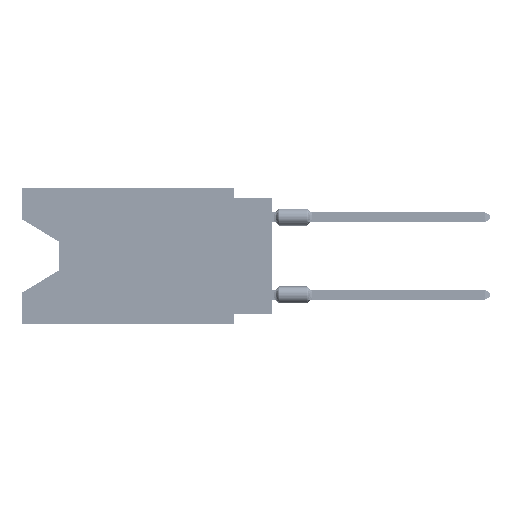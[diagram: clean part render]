
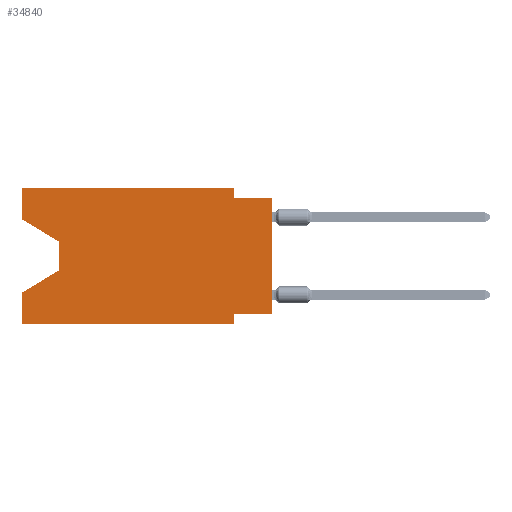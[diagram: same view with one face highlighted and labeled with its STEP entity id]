
A CAD part, left-side view. The second image highlights one B-rep face of the part: STEP entity #34840.
In plain terms, the highlighted planar face has unit normal (-1, 0, 0).
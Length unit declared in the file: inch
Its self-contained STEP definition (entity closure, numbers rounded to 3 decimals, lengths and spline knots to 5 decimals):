
#2917 = EDGE_CURVE ( 'NONE', #40746, #31872, #32700, .T. ) ;
#4210 = DIRECTION ( 'NONE',  ( 0., -1., 0. ) ) ;
#5944 = EDGE_CURVE ( 'NONE', #54752, #25376, #94050, .T. ) ;
#7796 = VECTOR ( 'NONE', #87289, 39.37008 ) ;
#8066 = LINE ( 'NONE', #54442, #36080 ) ;
#8804 = VECTOR ( 'NONE', #32441, 39.37008 ) ;
#9077 = AXIS2_PLACEMENT_3D ( 'NONE', #31439, #46383, #77770 ) ;
#9182 = EDGE_CURVE ( 'NONE', #25376, #62646, #38367, .T. ) ;
#9952 = CARTESIAN_POINT ( 'NONE',  ( 0., 0.55, -0.138 ) ) ;
#14926 = CARTESIAN_POINT ( 'NONE',  ( 0., 0.1, 0. ) ) ;
#15243 = CARTESIAN_POINT ( 'NONE',  ( 0., 0.645, 0. ) ) ;
#15249 = VECTOR ( 'NONE', #76084, 39.37008 ) ;
#16637 = CARTESIAN_POINT ( 'NONE',  ( 0., 0.645, -0.08025 ) ) ;
#17325 = CARTESIAN_POINT ( 'NONE',  ( 0., 0.645, -0.08025 ) ) ;
#18163 = DIRECTION ( 'NONE',  ( 0., -1., 0. ) ) ;
#21013 = EDGE_CURVE ( 'NONE', #54752, #31872, #58506, .T. ) ;
#22314 = EDGE_LOOP ( 'NONE', ( #92691, #84262, #61048, #60642, #31678, #40037, #41225, #31045, #81956, #97282, #42760, #35974 ) ) ;
#22325 = VECTOR ( 'NONE', #37398, 39.37008 ) ;
#24313 = EDGE_CURVE ( 'NONE', #33662, #62646, #78495, .T. ) ;
#24497 = EDGE_CURVE ( 'NONE', #43538, #70714, #51035, .T. ) ;
#24765 = CARTESIAN_POINT ( 'NONE',  ( 0., 0., -0.025 ) ) ;
#25376 = VERTEX_POINT ( 'NONE', #73224 ) ;
#29105 = CARTESIAN_POINT ( 'NONE',  ( 0., 0.645, 0. ) ) ;
#29898 = CARTESIAN_POINT ( 'NONE',  ( 0., 0.1, -0.35 ) ) ;
#30794 = EDGE_CURVE ( 'NONE', #33662, #82542, #83572, .T. ) ;
#31045 = ORIENTED_EDGE ( 'NONE', *, *, #21013, .T. ) ;
#31439 = CARTESIAN_POINT ( 'NONE',  ( 0., 0.645, 0. ) ) ;
#31678 = ORIENTED_EDGE ( 'NONE', *, *, #24313, .T. ) ;
#31872 = VERTEX_POINT ( 'NONE', #24765 ) ;
#32030 = EDGE_CURVE ( 'NONE', #59924, #82542, #8066, .T. ) ;
#32441 = DIRECTION ( 'NONE',  ( 0., 0., -1. ) ) ;
#32700 = LINE ( 'NONE', #79527, #45720 ) ;
#33120 = CARTESIAN_POINT ( 'NONE',  ( 0., 0.1, -0.35 ) ) ;
#33662 = VERTEX_POINT ( 'NONE', #46853 ) ;
#34840 = ADVANCED_FACE ( 'NONE', ( #84789 ), #75825, .F. ) ;
#35974 = ORIENTED_EDGE ( 'NONE', *, *, #92312, .F. ) ;
#36080 = VECTOR ( 'NONE', #91859, 39.37008 ) ;
#37398 = DIRECTION ( 'NONE',  ( 0., 0., -1. ) ) ;
#37876 = VECTOR ( 'NONE', #52776, 39.37008 ) ;
#38367 = LINE ( 'NONE', #29898, #22325 ) ;
#39634 = CARTESIAN_POINT ( 'NONE',  ( 0., 0.645, -0.35 ) ) ;
#40037 = ORIENTED_EDGE ( 'NONE', *, *, #9182, .F. ) ;
#40746 = VERTEX_POINT ( 'NONE', #66315 ) ;
#41220 = VECTOR ( 'NONE', #72580, 39.37008 ) ;
#41225 = ORIENTED_EDGE ( 'NONE', *, *, #5944, .F. ) ;
#42760 = ORIENTED_EDGE ( 'NONE', *, *, #24497, .F. ) ;
#43538 = VERTEX_POINT ( 'NONE', #73328 ) ;
#44368 = DIRECTION ( 'NONE',  ( 0., 0., -1. ) ) ;
#44512 = DIRECTION ( 'NONE',  ( 0., 0., 1. ) ) ;
#45720 = VECTOR ( 'NONE', #4210, 39.37008 ) ;
#45788 = LINE ( 'NONE', #68221, #37876 ) ;
#46383 = DIRECTION ( 'NONE',  ( 1., 0., 0. ) ) ;
#46853 = CARTESIAN_POINT ( 'NONE',  ( 0., 0.645, -0.35 ) ) ;
#49432 = VECTOR ( 'NONE', #44512, 39.37008 ) ;
#51035 = LINE ( 'NONE', #29105, #84973 ) ;
#52776 = DIRECTION ( 'NONE',  ( 0., 0., 1. ) ) ;
#54442 = CARTESIAN_POINT ( 'NONE',  ( 0., 0.55, -0.212 ) ) ;
#54752 = VERTEX_POINT ( 'NONE', #70514 ) ;
#54760 = CARTESIAN_POINT ( 'NONE',  ( 0., 0.645, -0.26975 ) ) ;
#57142 = VECTOR ( 'NONE', #44368, 39.37008 ) ;
#58137 = CARTESIAN_POINT ( 'NONE',  ( 0., 0., -0.325 ) ) ;
#58506 = LINE ( 'NONE', #90395, #49432 ) ;
#59317 = CARTESIAN_POINT ( 'NONE',  ( 0., 0.55, -0.212 ) ) ;
#59924 = VERTEX_POINT ( 'NONE', #59317 ) ;
#60642 = ORIENTED_EDGE ( 'NONE', *, *, #30794, .F. ) ;
#61048 = ORIENTED_EDGE ( 'NONE', *, *, #32030, .T. ) ;
#62646 = VERTEX_POINT ( 'NONE', #33120 ) ;
#63322 = LINE ( 'NONE', #9952, #8804 ) ;
#64245 = VECTOR ( 'NONE', #18163, 39.37008 ) ;
#65480 = DIRECTION ( 'NONE',  ( 0., -1., 0. ) ) ;
#66315 = CARTESIAN_POINT ( 'NONE',  ( 0., 0.1, -0.025 ) ) ;
#68221 = CARTESIAN_POINT ( 'NONE',  ( 0., 0.645, 0. ) ) ;
#68764 = EDGE_CURVE ( 'NONE', #95867, #59924, #63322, .T. ) ;
#70514 = CARTESIAN_POINT ( 'NONE',  ( 0., 0., -0.325 ) ) ;
#70714 = VERTEX_POINT ( 'NONE', #92053 ) ;
#72301 = LINE ( 'NONE', #16637, #7796 ) ;
#72580 = DIRECTION ( 'NONE',  ( 0., 1., 0. ) ) ;
#73224 = CARTESIAN_POINT ( 'NONE',  ( 0., 0.1, -0.325 ) ) ;
#73328 = CARTESIAN_POINT ( 'NONE',  ( 0., 0.645, 0. ) ) ;
#74623 = EDGE_CURVE ( 'NONE', #92492, #95867, #72301, .T. ) ;
#74801 = EDGE_CURVE ( 'NONE', #70714, #40746, #89759, .T. ) ;
#75825 = PLANE ( 'NONE',  #9077 ) ;
#76084 = DIRECTION ( 'NONE',  ( 0., 0., 1. ) ) ;
#77770 = DIRECTION ( 'NONE',  ( 0., 0., -1. ) ) ;
#78495 = LINE ( 'NONE', #39634, #64245 ) ;
#79527 = CARTESIAN_POINT ( 'NONE',  ( 0., 0., -0.025 ) ) ;
#79742 = CARTESIAN_POINT ( 'NONE',  ( 0., 0.55, -0.138 ) ) ;
#81956 = ORIENTED_EDGE ( 'NONE', *, *, #2917, .F. ) ;
#82542 = VERTEX_POINT ( 'NONE', #54760 ) ;
#83572 = LINE ( 'NONE', #15243, #15249 ) ;
#84262 = ORIENTED_EDGE ( 'NONE', *, *, #68764, .T. ) ;
#84789 = FACE_OUTER_BOUND ( 'NONE', #22314, .T. ) ;
#84973 = VECTOR ( 'NONE', #65480, 39.37008 ) ;
#87289 = DIRECTION ( 'NONE',  ( 0., -0.855, -0.519 ) ) ;
#89759 = LINE ( 'NONE', #14926, #57142 ) ;
#90395 = CARTESIAN_POINT ( 'NONE',  ( 0., 0., 0. ) ) ;
#91859 = DIRECTION ( 'NONE',  ( 0., 0.855, -0.519 ) ) ;
#92053 = CARTESIAN_POINT ( 'NONE',  ( 0., 0.1, 0. ) ) ;
#92312 = EDGE_CURVE ( 'NONE', #92492, #43538, #45788, .T. ) ;
#92492 = VERTEX_POINT ( 'NONE', #17325 ) ;
#92691 = ORIENTED_EDGE ( 'NONE', *, *, #74623, .T. ) ;
#94050 = LINE ( 'NONE', #58137, #41220 ) ;
#95867 = VERTEX_POINT ( 'NONE', #79742 ) ;
#97282 = ORIENTED_EDGE ( 'NONE', *, *, #74801, .F. ) ;
